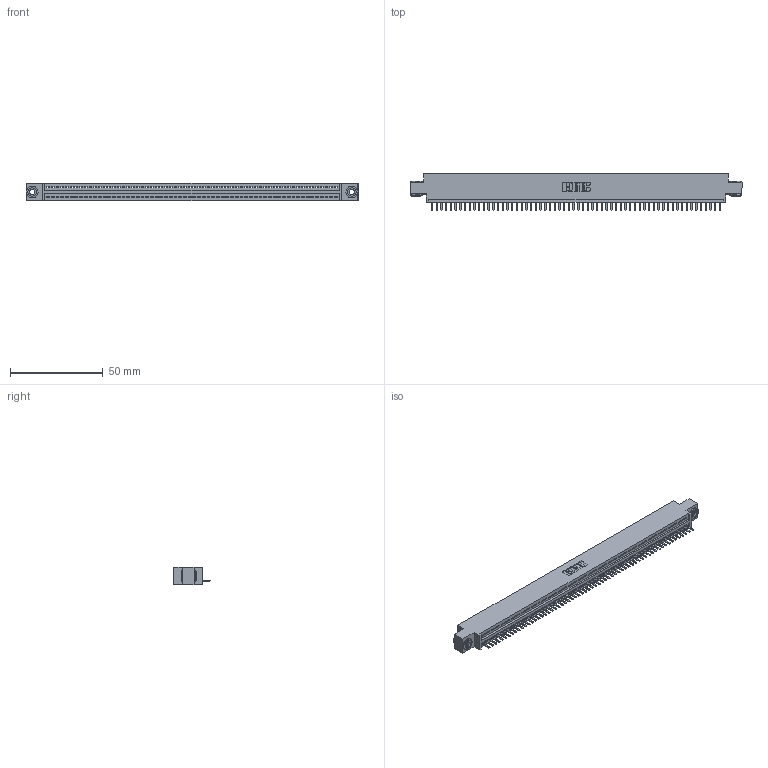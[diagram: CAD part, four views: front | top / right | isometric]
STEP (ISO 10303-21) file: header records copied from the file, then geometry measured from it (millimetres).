
FILE_DESCRIPTION (( 'STEP AP203' ), '1' );
FILE_NAME ('345-062-520-603.STEP', '2019-10-11T04:44:36', ( '' ), ( '' ), 'SwSTEP 2.0', 'SolidWorks 2016', '' );
FILE_SCHEMA (( 'CONFIG_CONTROL_DESIGN' ));
Length unit declared in the file: inch
Products named in the file (4): 345-250-002_345-250-002-102; 345-062-520-603; 345-292-001_345-293-120; 345 Part_0.170 Offset - 0.156 Dia-TH
Assembly tree (65 placements, depth 2):
  345-062-520-603
    345 Part_0.170 Offset - 0.156 Dia-TH
    345-292-001_345-293-120  x62
    345-250-002_345-250-002-102  x2
Bounding box: 178.69 x 19.68 x 9.4 mm (x, y, z)
Volume: 16863.6 mm3; surface area: 22439.6 mm2
Topology: 65 solids, 65 shells, 4012 faces, 11837 edges, 7722 vertices
Faces by surface type: plane 2698, cylinder 1306, cone 8
Entity records: 44866 total; most frequent: CARTESIAN_POINT 7761, ORIENTED_EDGE 7738, DIRECTION 6767, EDGE_CURVE 3869, LINE 3461, VECTOR 3461, VERTEX_POINT 2574, AXIS2_PLACEMENT_3D 1653
